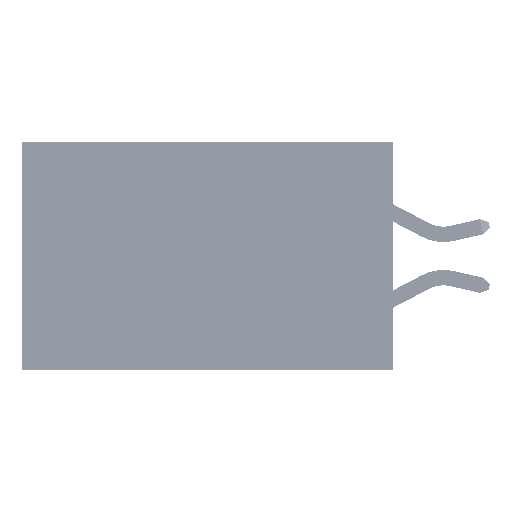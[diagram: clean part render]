
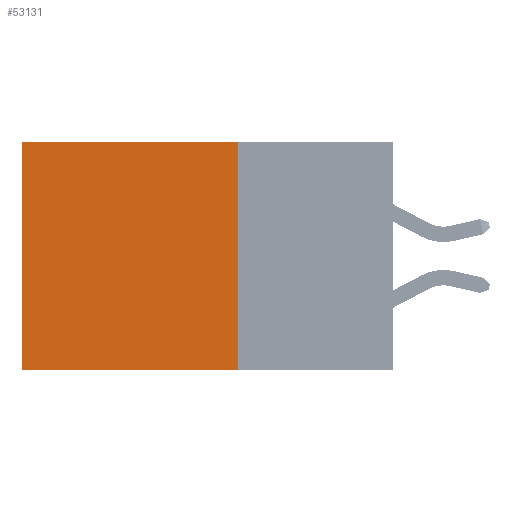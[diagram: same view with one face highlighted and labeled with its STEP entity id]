
A CAD part, left-side view. The second image highlights one B-rep face of the part: STEP entity #53131.
In plain terms, the highlighted planar face has unit normal (-1, 0, 0).
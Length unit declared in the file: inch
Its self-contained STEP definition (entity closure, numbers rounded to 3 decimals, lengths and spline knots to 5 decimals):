
#472 = VERTEX_POINT ( 'NONE', #33960 ) ;
#3210 = ORIENTED_EDGE ( 'NONE', *, *, #37203, .F. ) ;
#5826 = VERTEX_POINT ( 'NONE', #27218 ) ;
#6235 = AXIS2_PLACEMENT_3D ( 'NONE', #32149, #44464, #19937 ) ;
#6613 = VECTOR ( 'NONE', #45949, 39.37008 ) ;
#13442 = DIRECTION ( 'NONE',  ( 0., 0., -1. ) ) ;
#14838 = EDGE_CURVE ( 'NONE', #5826, #39040, #43631, .T. ) ;
#15780 = PLANE ( 'NONE',  #6235 ) ;
#15913 = ORIENTED_EDGE ( 'NONE', *, *, #25977, .F. ) ;
#17439 = CARTESIAN_POINT ( 'NONE',  ( 0.2875, 0.25, 0. ) ) ;
#19031 = ORIENTED_EDGE ( 'NONE', *, *, #14838, .T. ) ;
#19937 = DIRECTION ( 'NONE',  ( 0., 0., -1. ) ) ;
#20394 = LINE ( 'NONE', #17439, #39634 ) ;
#21430 = CARTESIAN_POINT ( 'NONE',  ( 0.2875, 0.6, 0. ) ) ;
#23258 = FACE_OUTER_BOUND ( 'NONE', #25418, .T. ) ;
#23617 = DIRECTION ( 'NONE',  ( 0., 1., 0. ) ) ;
#23662 = ORIENTED_EDGE ( 'NONE', *, *, #29230, .T. ) ;
#24594 = DIRECTION ( 'NONE',  ( 0., 1., 0. ) ) ;
#25418 = EDGE_LOOP ( 'NONE', ( #23662, #3210, #15913, #19031 ) ) ;
#25977 = EDGE_CURVE ( 'NONE', #5826, #26737, #20394, .T. ) ;
#26016 = CARTESIAN_POINT ( 'NONE',  ( 0.2875, 0.25, -0.37 ) ) ;
#26737 = VERTEX_POINT ( 'NONE', #26016 ) ;
#27218 = CARTESIAN_POINT ( 'NONE',  ( 0.2875, 0.25, 0. ) ) ;
#29230 = EDGE_CURVE ( 'NONE', #39040, #472, #39449, .T. ) ;
#31849 = LINE ( 'NONE', #32836, #51036 ) ;
#32149 = CARTESIAN_POINT ( 'NONE',  ( 0.2875, 0.25, 0. ) ) ;
#32836 = CARTESIAN_POINT ( 'NONE',  ( 0.2875, 0.25, -0.37 ) ) ;
#33960 = CARTESIAN_POINT ( 'NONE',  ( 0.2875, 0.6, -0.37 ) ) ;
#37203 = EDGE_CURVE ( 'NONE', #26737, #472, #31849, .T. ) ;
#39040 = VERTEX_POINT ( 'NONE', #44598 ) ;
#39449 = LINE ( 'NONE', #21430, #6613 ) ;
#39634 = VECTOR ( 'NONE', #13442, 39.37008 ) ;
#39905 = CARTESIAN_POINT ( 'NONE',  ( 0.2875, 0.25, 0. ) ) ;
#43631 = LINE ( 'NONE', #39905, #51951 ) ;
#44464 = DIRECTION ( 'NONE',  ( 1., 0., 0. ) ) ;
#44598 = CARTESIAN_POINT ( 'NONE',  ( 0.2875, 0.6, 0. ) ) ;
#45949 = DIRECTION ( 'NONE',  ( 0., 0., -1. ) ) ;
#51036 = VECTOR ( 'NONE', #24594, 39.37008 ) ;
#51951 = VECTOR ( 'NONE', #23617, 39.37008 ) ;
#53131 = ADVANCED_FACE ( 'NONE', ( #23258 ), #15780, .F. ) ;
